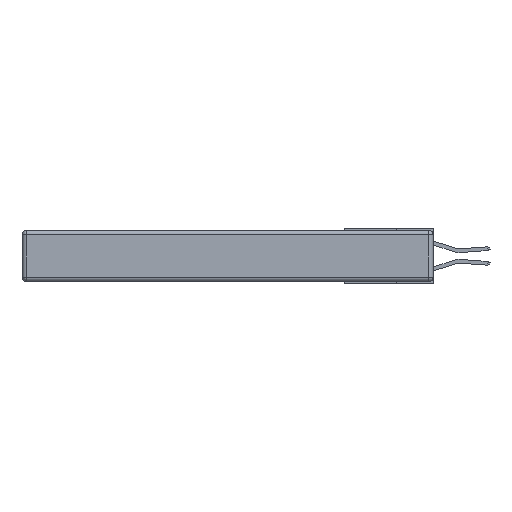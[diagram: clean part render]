
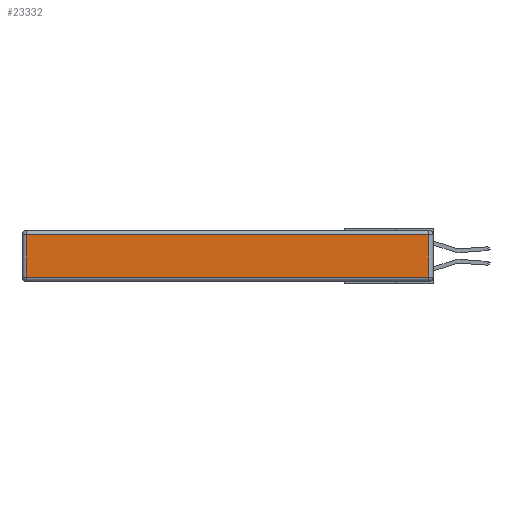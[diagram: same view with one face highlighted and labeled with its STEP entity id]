
A CAD part, left-side view. The second image highlights one B-rep face of the part: STEP entity #23332.
In plain terms, the highlighted planar face has unit normal (-1, 0, 0).
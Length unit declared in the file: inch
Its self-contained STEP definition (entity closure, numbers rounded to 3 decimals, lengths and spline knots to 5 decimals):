
#2020 = EDGE_CURVE ( 'NONE', #20949, #27384, #7607, .T. ) ;
#2972 = CARTESIAN_POINT ( 'NONE',  ( 0., 2.72, -0.343 ) ) ;
#2998 = VECTOR ( 'NONE', #11267, 39.37008 ) ;
#4130 = CARTESIAN_POINT ( 'NONE',  ( 0., 2.72, -0.03 ) ) ;
#4453 = LINE ( 'NONE', #23114, #16155 ) ;
#4751 = EDGE_CURVE ( 'NONE', #27384, #24856, #4453, .T. ) ;
#7607 = LINE ( 'NONE', #18718, #14015 ) ;
#8463 = VERTEX_POINT ( 'NONE', #23557 ) ;
#8681 = LINE ( 'NONE', #13340, #2998 ) ;
#9218 = DIRECTION ( 'NONE',  ( 0., 0., -1. ) ) ;
#9947 = DIRECTION ( 'NONE',  ( 0., 0., 1. ) ) ;
#10162 = ORIENTED_EDGE ( 'NONE', *, *, #2020, .T. ) ;
#10546 = AXIS2_PLACEMENT_3D ( 'NONE', #13384, #21960, #17560 ) ;
#11267 = DIRECTION ( 'NONE',  ( 0., -1., 0. ) ) ;
#12036 = EDGE_CURVE ( 'NONE', #24856, #8463, #12660, .T. ) ;
#12660 = LINE ( 'NONE', #2972, #20343 ) ;
#13340 = CARTESIAN_POINT ( 'NONE',  ( 0., 0., -0.313 ) ) ;
#13384 = CARTESIAN_POINT ( 'NONE',  ( 0., 0., -0.343 ) ) ;
#14015 = VECTOR ( 'NONE', #9947, 39.37008 ) ;
#16014 = ORIENTED_EDGE ( 'NONE', *, *, #17219, .T. ) ;
#16155 = VECTOR ( 'NONE', #27317, 39.37008 ) ;
#16826 = FACE_OUTER_BOUND ( 'NONE', #19759, .T. ) ;
#17219 = EDGE_CURVE ( 'NONE', #8463, #20949, #8681, .T. ) ;
#17560 = DIRECTION ( 'NONE',  ( 0., 0., 1. ) ) ;
#17910 = ORIENTED_EDGE ( 'NONE', *, *, #12036, .T. ) ;
#18718 = CARTESIAN_POINT ( 'NONE',  ( 0., 0.03, -0.343 ) ) ;
#19759 = EDGE_LOOP ( 'NONE', ( #16014, #10162, #22191, #17910 ) ) ;
#20343 = VECTOR ( 'NONE', #9218, 39.37008 ) ;
#20461 = CARTESIAN_POINT ( 'NONE',  ( 0., 0.03, -0.03 ) ) ;
#20949 = VERTEX_POINT ( 'NONE', #23881 ) ;
#21960 = DIRECTION ( 'NONE',  ( -1., 0., 0. ) ) ;
#22191 = ORIENTED_EDGE ( 'NONE', *, *, #4751, .T. ) ;
#23114 = CARTESIAN_POINT ( 'NONE',  ( 0., 2.75, -0.03 ) ) ;
#23332 = ADVANCED_FACE ( 'NONE', ( #16826 ), #26052, .T. ) ;
#23557 = CARTESIAN_POINT ( 'NONE',  ( 0., 2.72, -0.313 ) ) ;
#23881 = CARTESIAN_POINT ( 'NONE',  ( 0., 0.03, -0.313 ) ) ;
#24856 = VERTEX_POINT ( 'NONE', #4130 ) ;
#26052 = PLANE ( 'NONE',  #10546 ) ;
#27317 = DIRECTION ( 'NONE',  ( 0., 1., 0. ) ) ;
#27384 = VERTEX_POINT ( 'NONE', #20461 ) ;
